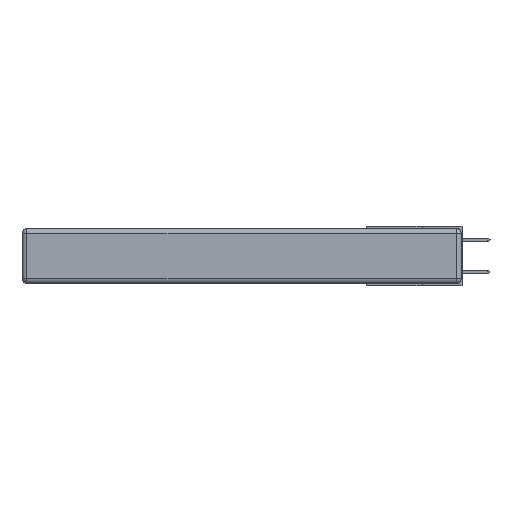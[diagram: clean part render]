
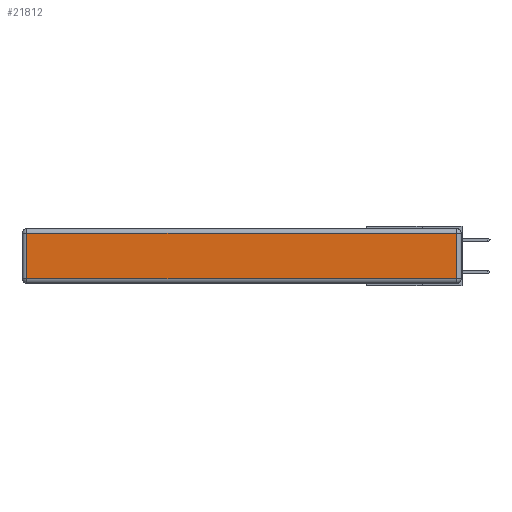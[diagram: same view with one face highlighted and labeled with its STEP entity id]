
A CAD part, left-side view. The second image highlights one B-rep face of the part: STEP entity #21812.
In plain terms, the highlighted planar face has unit normal (-1, 0, 0).
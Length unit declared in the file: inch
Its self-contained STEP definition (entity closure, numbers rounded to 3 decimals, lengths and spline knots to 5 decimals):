
#619 = VERTEX_POINT ( 'NONE', #15738 ) ;
#798 = CARTESIAN_POINT ( 'NONE',  ( 0., 0.03, -0.343 ) ) ;
#1577 = DIRECTION ( 'NONE',  ( 0., 1., 0. ) ) ;
#1937 = ORIENTED_EDGE ( 'NONE', *, *, #4507, .T. ) ;
#2033 = DIRECTION ( 'NONE',  ( 0., -1., 0. ) ) ;
#2769 = VERTEX_POINT ( 'NONE', #11521 ) ;
#2962 = VECTOR ( 'NONE', #4392, 39.37008 ) ;
#3126 = ORIENTED_EDGE ( 'NONE', *, *, #18625, .T. ) ;
#3194 = DIRECTION ( 'NONE',  ( -1., 0., 0. ) ) ;
#4392 = DIRECTION ( 'NONE',  ( 0., 0., 1. ) ) ;
#4507 = EDGE_CURVE ( 'NONE', #2769, #619, #8060, .T. ) ;
#4652 = AXIS2_PLACEMENT_3D ( 'NONE', #8589, #3194, #11925 ) ;
#5273 = VECTOR ( 'NONE', #1577, 39.37008 ) ;
#5442 = LINE ( 'NONE', #14951, #6211 ) ;
#6211 = VECTOR ( 'NONE', #11627, 39.37008 ) ;
#6732 = PLANE ( 'NONE',  #4652 ) ;
#7727 = EDGE_CURVE ( 'NONE', #619, #15614, #7979, .T. ) ;
#7979 = LINE ( 'NONE', #798, #2962 ) ;
#8060 = LINE ( 'NONE', #18919, #17058 ) ;
#8589 = CARTESIAN_POINT ( 'NONE',  ( 0., 0., -0.343 ) ) ;
#10848 = LINE ( 'NONE', #20080, #5273 ) ;
#11521 = CARTESIAN_POINT ( 'NONE',  ( 0., 2.72, -0.313 ) ) ;
#11627 = DIRECTION ( 'NONE',  ( 0., 0., -1. ) ) ;
#11925 = DIRECTION ( 'NONE',  ( 0., 0., 1. ) ) ;
#13537 = ORIENTED_EDGE ( 'NONE', *, *, #7727, .T. ) ;
#13830 = EDGE_CURVE ( 'NONE', #16799, #2769, #5442, .T. ) ;
#14951 = CARTESIAN_POINT ( 'NONE',  ( 0., 2.72, -0.343 ) ) ;
#15614 = VERTEX_POINT ( 'NONE', #20162 ) ;
#15738 = CARTESIAN_POINT ( 'NONE',  ( 0., 0.03, -0.313 ) ) ;
#16735 = ORIENTED_EDGE ( 'NONE', *, *, #13830, .T. ) ;
#16799 = VERTEX_POINT ( 'NONE', #21585 ) ;
#17058 = VECTOR ( 'NONE', #2033, 39.37008 ) ;
#18625 = EDGE_CURVE ( 'NONE', #15614, #16799, #10848, .T. ) ;
#18919 = CARTESIAN_POINT ( 'NONE',  ( 0., 0., -0.313 ) ) ;
#18969 = EDGE_LOOP ( 'NONE', ( #1937, #13537, #3126, #16735 ) ) ;
#20080 = CARTESIAN_POINT ( 'NONE',  ( 0., 2.75, -0.03 ) ) ;
#20162 = CARTESIAN_POINT ( 'NONE',  ( 0., 0.03, -0.03 ) ) ;
#20316 = FACE_OUTER_BOUND ( 'NONE', #18969, .T. ) ;
#21585 = CARTESIAN_POINT ( 'NONE',  ( 0., 2.72, -0.03 ) ) ;
#21812 = ADVANCED_FACE ( 'NONE', ( #20316 ), #6732, .T. ) ;
